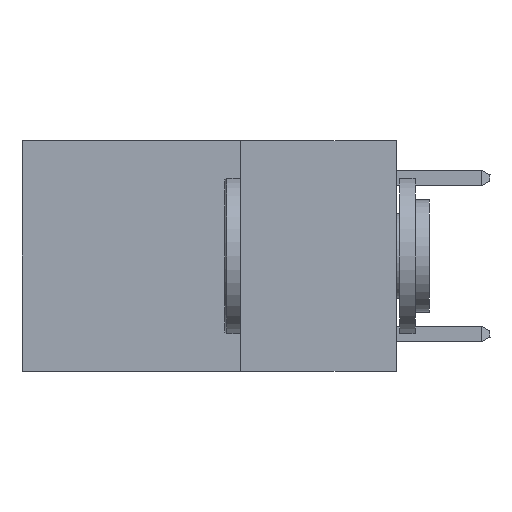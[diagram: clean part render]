
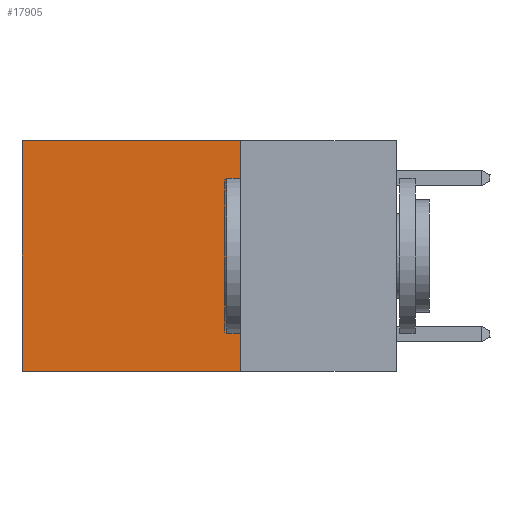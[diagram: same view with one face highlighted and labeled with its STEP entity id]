
A CAD part, left-side view. The second image highlights one B-rep face of the part: STEP entity #17905.
In plain terms, the highlighted planar face has unit normal (-1, 0, 0).
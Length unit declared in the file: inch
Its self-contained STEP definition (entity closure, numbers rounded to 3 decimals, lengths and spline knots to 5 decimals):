
#466 = EDGE_CURVE ( 'NONE', #8156, #8389, #13249, .T. ) ;
#972 = CARTESIAN_POINT ( 'NONE',  ( 0.2625, 0.25, 0. ) ) ;
#994 = DIRECTION ( 'NONE',  ( 0., 0., -1. ) ) ;
#1353 = DIRECTION ( 'NONE',  ( 0., 0., -1. ) ) ;
#1700 = VECTOR ( 'NONE', #6563, 39.37008 ) ;
#2466 = DIRECTION ( 'NONE',  ( 0., 0., -1. ) ) ;
#3598 = EDGE_CURVE ( 'NONE', #12193, #6227, #6366, .T. ) ;
#4087 = CARTESIAN_POINT ( 'NONE',  ( 0.2625, 0.25, 0. ) ) ;
#4658 = CARTESIAN_POINT ( 'NONE',  ( 0.2625, 0.25, 0. ) ) ;
#5282 = ORIENTED_EDGE ( 'NONE', *, *, #3598, .F. ) ;
#5847 = DIRECTION ( 'NONE',  ( 1., 0., 0. ) ) ;
#6227 = VERTEX_POINT ( 'NONE', #12674 ) ;
#6366 = LINE ( 'NONE', #18662, #1700 ) ;
#6553 = EDGE_CURVE ( 'NONE', #8389, #6227, #11841, .T. ) ;
#6563 = DIRECTION ( 'NONE',  ( 0., 1., 0. ) ) ;
#6648 = ORIENTED_EDGE ( 'NONE', *, *, #466, .T. ) ;
#6701 = ORIENTED_EDGE ( 'NONE', *, *, #6984, .F. ) ;
#6984 = EDGE_CURVE ( 'NONE', #8156, #12193, #8698, .T. ) ;
#7175 = ORIENTED_EDGE ( 'NONE', *, *, #6553, .T. ) ;
#7739 = CARTESIAN_POINT ( 'NONE',  ( 0.2625, 0.25, -0.37 ) ) ;
#8156 = VERTEX_POINT ( 'NONE', #19082 ) ;
#8389 = VERTEX_POINT ( 'NONE', #19363 ) ;
#8698 = LINE ( 'NONE', #972, #12175 ) ;
#11841 = LINE ( 'NONE', #17802, #12158 ) ;
#12158 = VECTOR ( 'NONE', #994, 39.37008 ) ;
#12175 = VECTOR ( 'NONE', #2466, 39.37008 ) ;
#12193 = VERTEX_POINT ( 'NONE', #7739 ) ;
#12196 = PLANE ( 'NONE',  #16758 ) ;
#12674 = CARTESIAN_POINT ( 'NONE',  ( 0.2625, 0.6, -0.37 ) ) ;
#13249 = LINE ( 'NONE', #4087, #18335 ) ;
#16185 = EDGE_LOOP ( 'NONE', ( #7175, #5282, #6701, #6648 ) ) ;
#16758 = AXIS2_PLACEMENT_3D ( 'NONE', #4658, #5847, #1353 ) ;
#17419 = DIRECTION ( 'NONE',  ( 0., 1., 0. ) ) ;
#17802 = CARTESIAN_POINT ( 'NONE',  ( 0.2625, 0.6, 0. ) ) ;
#17905 = ADVANCED_FACE ( 'NONE', ( #18039 ), #12196, .F. ) ;
#18039 = FACE_OUTER_BOUND ( 'NONE', #16185, .T. ) ;
#18335 = VECTOR ( 'NONE', #17419, 39.37008 ) ;
#18662 = CARTESIAN_POINT ( 'NONE',  ( 0.2625, 0.25, -0.37 ) ) ;
#19082 = CARTESIAN_POINT ( 'NONE',  ( 0.2625, 0.25, 0. ) ) ;
#19363 = CARTESIAN_POINT ( 'NONE',  ( 0.2625, 0.6, 0. ) ) ;
